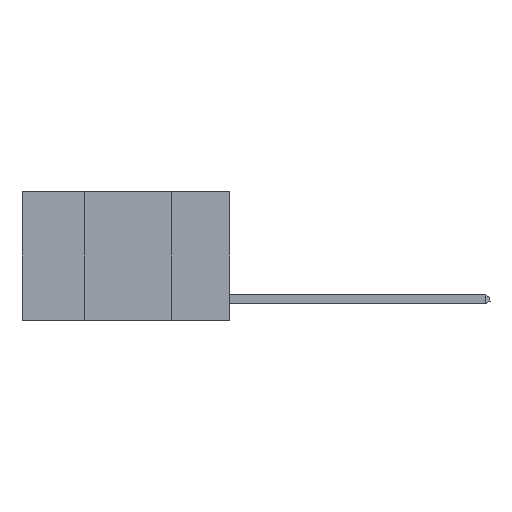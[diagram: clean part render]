
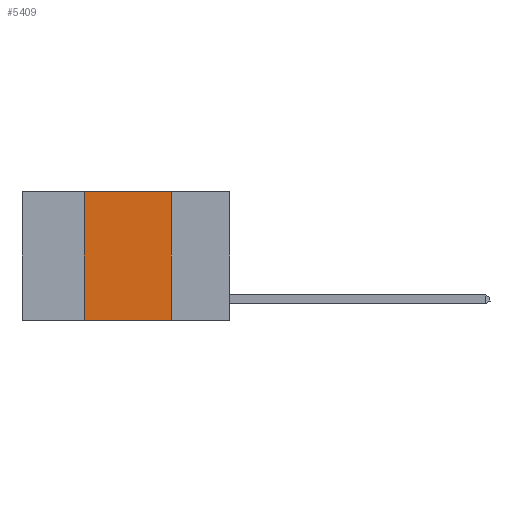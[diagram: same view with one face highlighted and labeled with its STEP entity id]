
A CAD part, left-side view. The second image highlights one B-rep face of the part: STEP entity #5409.
In plain terms, the highlighted planar face has unit normal (-1, 0, 0).
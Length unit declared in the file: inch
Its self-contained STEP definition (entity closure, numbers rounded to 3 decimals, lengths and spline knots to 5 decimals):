
#389 = CARTESIAN_POINT ( 'NONE',  ( 0., 0.17, 0. ) ) ;
#1282 = ORIENTED_EDGE ( 'NONE', *, *, #2052, .F. ) ;
#1344 = DIRECTION ( 'NONE',  ( 0., 0., 1. ) ) ;
#2052 = EDGE_CURVE ( 'NONE', #9768, #9759, #5951, .T. ) ;
#2468 = ORIENTED_EDGE ( 'NONE', *, *, #3118, .F. ) ;
#2647 = DIRECTION ( 'NONE',  ( 1., 0., 0. ) ) ;
#3118 = EDGE_CURVE ( 'NONE', #7639, #7178, #7653, .T. ) ;
#3179 = VECTOR ( 'NONE', #9313, 39.37008 ) ;
#3433 = VECTOR ( 'NONE', #1344, 39.37008 ) ;
#3624 = EDGE_CURVE ( 'NONE', #7639, #9759, #9362, .T. ) ;
#4012 = CARTESIAN_POINT ( 'NONE',  ( 0., 0.6, -0.37 ) ) ;
#4065 = FACE_OUTER_BOUND ( 'NONE', #5487, .T. ) ;
#4781 = CARTESIAN_POINT ( 'NONE',  ( 0., 0.42, 0. ) ) ;
#5128 = CARTESIAN_POINT ( 'NONE',  ( 0., 0.17, 0. ) ) ;
#5409 = ADVANCED_FACE ( 'NONE', ( #4065 ), #7454, .F. ) ;
#5487 = EDGE_LOOP ( 'NONE', ( #1282, #9325, #2468, #9965 ) ) ;
#5515 = EDGE_CURVE ( 'NONE', #7178, #9768, #7918, .T. ) ;
#5951 = LINE ( 'NONE', #5128, #7674 ) ;
#6463 = CARTESIAN_POINT ( 'NONE',  ( 0., 0.42, -0.37 ) ) ;
#6489 = AXIS2_PLACEMENT_3D ( 'NONE', #9608, #2647, #8151 ) ;
#6767 = DIRECTION ( 'NONE',  ( 0., 0., -1. ) ) ;
#6971 = DIRECTION ( 'NONE',  ( 0., -1., 0. ) ) ;
#7178 = VERTEX_POINT ( 'NONE', #4781 ) ;
#7454 = PLANE ( 'NONE',  #6489 ) ;
#7639 = VERTEX_POINT ( 'NONE', #6463 ) ;
#7653 = LINE ( 'NONE', #10098, #3433 ) ;
#7674 = VECTOR ( 'NONE', #6767, 39.37008 ) ;
#7918 = LINE ( 'NONE', #9934, #9677 ) ;
#8151 = DIRECTION ( 'NONE',  ( 0., 0., -1. ) ) ;
#9313 = DIRECTION ( 'NONE',  ( 0., -1., 0. ) ) ;
#9325 = ORIENTED_EDGE ( 'NONE', *, *, #5515, .F. ) ;
#9362 = LINE ( 'NONE', #4012, #3179 ) ;
#9608 = CARTESIAN_POINT ( 'NONE',  ( 0., 0.6, 0. ) ) ;
#9677 = VECTOR ( 'NONE', #6971, 39.37008 ) ;
#9759 = VERTEX_POINT ( 'NONE', #9762 ) ;
#9762 = CARTESIAN_POINT ( 'NONE',  ( 0., 0.17, -0.37 ) ) ;
#9768 = VERTEX_POINT ( 'NONE', #389 ) ;
#9934 = CARTESIAN_POINT ( 'NONE',  ( 0., 0.6, 0. ) ) ;
#9965 = ORIENTED_EDGE ( 'NONE', *, *, #3624, .T. ) ;
#10098 = CARTESIAN_POINT ( 'NONE',  ( 0., 0.42, 0. ) ) ;
